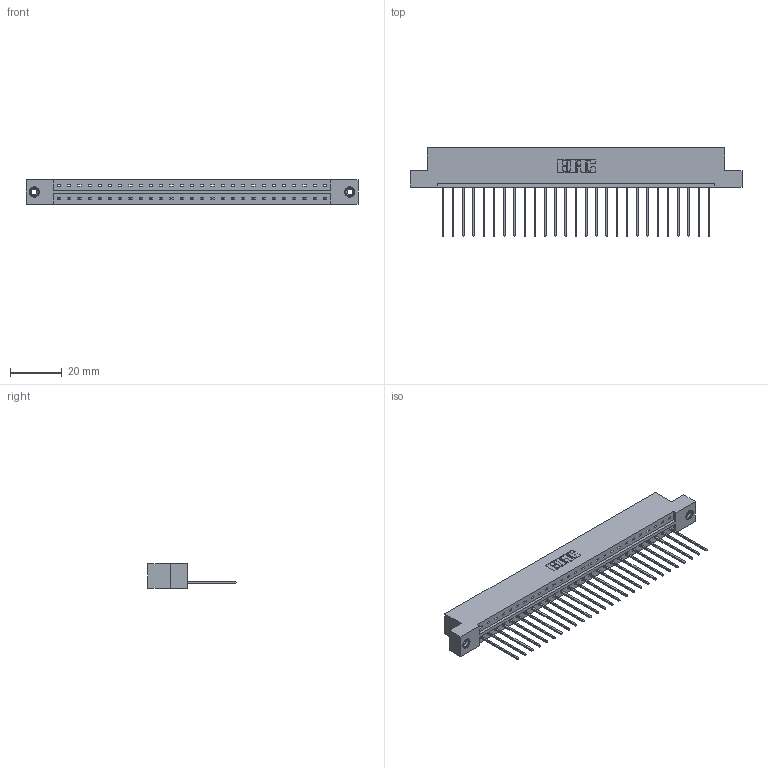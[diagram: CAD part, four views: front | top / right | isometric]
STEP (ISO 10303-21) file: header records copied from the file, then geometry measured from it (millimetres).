
FILE_DESCRIPTION (( 'STEP AP203' ), '1' );
FILE_NAME ('333-027-541-108.STEP', '2018-08-02T14:02:57', ( '' ), ( '' ), 'SwSTEP 2.0', 'SolidWorks 2016', '' );
FILE_SCHEMA (( 'CONFIG_CONTROL_DESIGN' ));
Length unit declared in the file: inch
Products named in the file (4): 345-250-001_345-250-003-102; 333-027-541-108; 333 Part_Flush - .156 Dia - TI; 345-292-001_345-293-141
Assembly tree (30 placements, depth 2):
  333-027-541-108
    333 Part_Flush - .156 Dia - TI
    345-292-001_345-293-141  x27
    345-250-001_345-250-003-102  x2
Bounding box: 128.52 x 34.3 x 9.4 mm (x, y, z)
Volume: 12886.7 mm3; surface area: 14417.9 mm2
Topology: 30 solids, 30 shells, 1740 faces, 5199 edges, 3422 vertices
Faces by surface type: plane 1236, cylinder 488, cone 12, torus 4
Entity records: 19650 total; most frequent: CARTESIAN_POINT 3374, ORIENTED_EDGE 3330, DIRECTION 2909, EDGE_CURVE 1665, LINE 1517, VECTOR 1517, VERTEX_POINT 1104, AXIS2_PLACEMENT_3D 696
